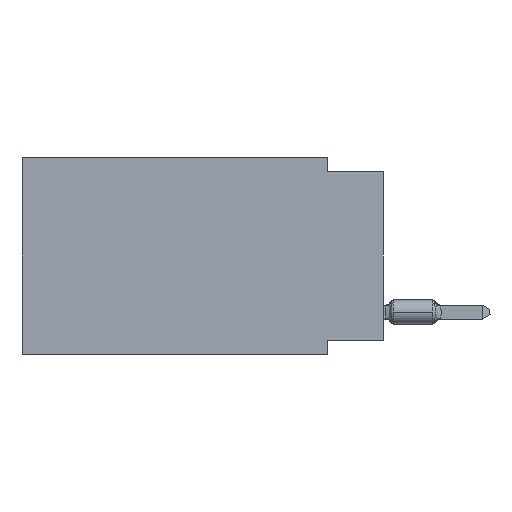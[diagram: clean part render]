
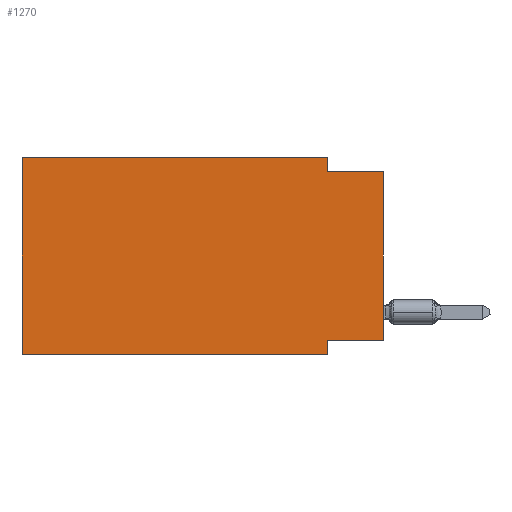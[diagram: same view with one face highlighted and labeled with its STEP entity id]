
A CAD part, left-side view. The second image highlights one B-rep face of the part: STEP entity #1270.
In plain terms, the highlighted planar face has unit normal (-1, 0, 0).
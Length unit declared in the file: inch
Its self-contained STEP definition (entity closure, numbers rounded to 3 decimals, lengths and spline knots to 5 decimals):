
#919 = FACE_OUTER_BOUND ( 'NONE', #6825, .T. ) ;
#1088 = DIRECTION ( 'NONE',  ( 0., -1., 0. ) ) ;
#1231 = DIRECTION ( 'NONE',  ( 0., 0., -1. ) ) ;
#1270 = ADVANCED_FACE ( 'NONE', ( #919 ), #24057, .F. ) ;
#2088 = EDGE_CURVE ( 'NONE', #18870, #2638, #3286, .T. ) ;
#2529 = LINE ( 'NONE', #20579, #25752 ) ;
#2578 = ORIENTED_EDGE ( 'NONE', *, *, #27152, .F. ) ;
#2638 = VERTEX_POINT ( 'NONE', #8216 ) ;
#2867 = LINE ( 'NONE', #11663, #6397 ) ;
#3286 = LINE ( 'NONE', #21947, #24250 ) ;
#3768 = DIRECTION ( 'NONE',  ( 0., 0., -1. ) ) ;
#4505 = VERTEX_POINT ( 'NONE', #16682 ) ;
#4552 = DIRECTION ( 'NONE',  ( 0., 0., 1. ) ) ;
#4846 = CARTESIAN_POINT ( 'NONE',  ( 0., 0.1, -0.325 ) ) ;
#4975 = VECTOR ( 'NONE', #29509, 39.37008 ) ;
#5143 = AXIS2_PLACEMENT_3D ( 'NONE', #19420, #17116, #1231 ) ;
#6086 = CARTESIAN_POINT ( 'NONE',  ( 0., 0.1, -0.35 ) ) ;
#6397 = VECTOR ( 'NONE', #21374, 39.37008 ) ;
#6792 = ORIENTED_EDGE ( 'NONE', *, *, #19312, .F. ) ;
#6824 = CARTESIAN_POINT ( 'NONE',  ( 0., 0., -0.325 ) ) ;
#6825 = EDGE_LOOP ( 'NONE', ( #14573, #16383, #12223, #9873, #28818, #21419, #2578, #6792 ) ) ;
#7934 = CARTESIAN_POINT ( 'NONE',  ( 0., 0., -0.025 ) ) ;
#7996 = EDGE_CURVE ( 'NONE', #20706, #4505, #2867, .T. ) ;
#8216 = CARTESIAN_POINT ( 'NONE',  ( 0., 0.1, -0.025 ) ) ;
#8231 = CARTESIAN_POINT ( 'NONE',  ( 0., 0.645, -0.35 ) ) ;
#8612 = VECTOR ( 'NONE', #3768, 39.37008 ) ;
#8834 = CARTESIAN_POINT ( 'NONE',  ( 0., 0., -0.325 ) ) ;
#9394 = EDGE_CURVE ( 'NONE', #2638, #10270, #26740, .T. ) ;
#9873 = ORIENTED_EDGE ( 'NONE', *, *, #22289, .F. ) ;
#10270 = VERTEX_POINT ( 'NONE', #17668 ) ;
#10276 = VECTOR ( 'NONE', #1088, 39.37008 ) ;
#10520 = EDGE_CURVE ( 'NONE', #20706, #28815, #2529, .T. ) ;
#10821 = CARTESIAN_POINT ( 'NONE',  ( 0., 0.645, 0. ) ) ;
#11340 = LINE ( 'NONE', #16718, #17795 ) ;
#11663 = CARTESIAN_POINT ( 'NONE',  ( 0., 0.645, -0.35 ) ) ;
#11979 = VERTEX_POINT ( 'NONE', #6824 ) ;
#12223 = ORIENTED_EDGE ( 'NONE', *, *, #2088, .F. ) ;
#14573 = ORIENTED_EDGE ( 'NONE', *, *, #17676, .T. ) ;
#15381 = VECTOR ( 'NONE', #15763, 39.37008 ) ;
#15763 = DIRECTION ( 'NONE',  ( 0., 1., 0. ) ) ;
#16383 = ORIENTED_EDGE ( 'NONE', *, *, #9394, .F. ) ;
#16682 = CARTESIAN_POINT ( 'NONE',  ( 0., 0.1, -0.35 ) ) ;
#16718 = CARTESIAN_POINT ( 'NONE',  ( 0., 0., 0. ) ) ;
#17116 = DIRECTION ( 'NONE',  ( 1., 0., 0. ) ) ;
#17668 = CARTESIAN_POINT ( 'NONE',  ( 0., 0., -0.025 ) ) ;
#17676 = EDGE_CURVE ( 'NONE', #11979, #10270, #11340, .T. ) ;
#17795 = VECTOR ( 'NONE', #4552, 39.37008 ) ;
#18526 = LINE ( 'NONE', #8834, #15381 ) ;
#18870 = VERTEX_POINT ( 'NONE', #26929 ) ;
#19312 = EDGE_CURVE ( 'NONE', #11979, #23875, #18526, .T. ) ;
#19420 = CARTESIAN_POINT ( 'NONE',  ( 0., 0.645, 0. ) ) ;
#20244 = DIRECTION ( 'NONE',  ( 0., 0., -1. ) ) ;
#20579 = CARTESIAN_POINT ( 'NONE',  ( 0., 0.645, 0. ) ) ;
#20706 = VERTEX_POINT ( 'NONE', #8231 ) ;
#21374 = DIRECTION ( 'NONE',  ( 0., -1., 0. ) ) ;
#21419 = ORIENTED_EDGE ( 'NONE', *, *, #7996, .T. ) ;
#21947 = CARTESIAN_POINT ( 'NONE',  ( 0., 0.1, 0. ) ) ;
#22289 = EDGE_CURVE ( 'NONE', #28815, #18870, #24832, .T. ) ;
#23875 = VERTEX_POINT ( 'NONE', #4846 ) ;
#24057 = PLANE ( 'NONE',  #5143 ) ;
#24250 = VECTOR ( 'NONE', #20244, 39.37008 ) ;
#24832 = LINE ( 'NONE', #10821, #10276 ) ;
#25752 = VECTOR ( 'NONE', #30128, 39.37008 ) ;
#26740 = LINE ( 'NONE', #7934, #4975 ) ;
#26929 = CARTESIAN_POINT ( 'NONE',  ( 0., 0.1, 0. ) ) ;
#26931 = CARTESIAN_POINT ( 'NONE',  ( 0., 0.645, 0. ) ) ;
#27152 = EDGE_CURVE ( 'NONE', #23875, #4505, #27212, .T. ) ;
#27212 = LINE ( 'NONE', #6086, #8612 ) ;
#28815 = VERTEX_POINT ( 'NONE', #26931 ) ;
#28818 = ORIENTED_EDGE ( 'NONE', *, *, #10520, .F. ) ;
#29509 = DIRECTION ( 'NONE',  ( 0., -1., 0. ) ) ;
#30128 = DIRECTION ( 'NONE',  ( 0., 0., 1. ) ) ;
